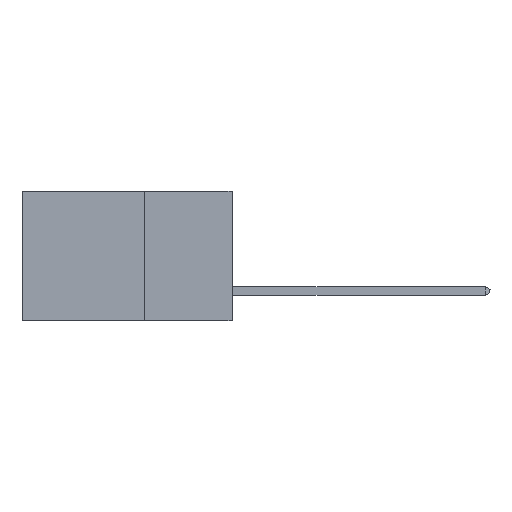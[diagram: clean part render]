
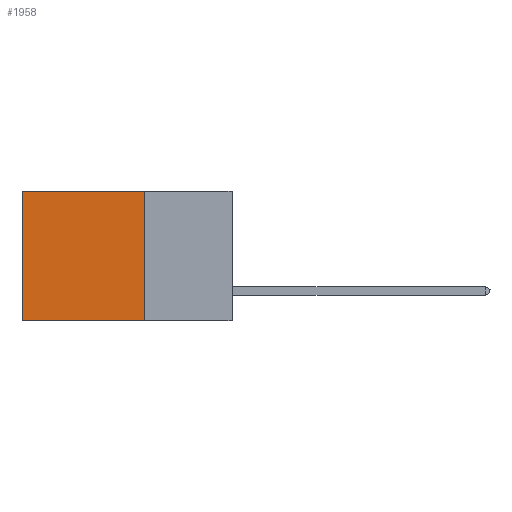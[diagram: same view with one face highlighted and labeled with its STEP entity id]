
A CAD part, left-side view. The second image highlights one B-rep face of the part: STEP entity #1958.
In plain terms, the highlighted planar face has unit normal (-1, 0, 0).
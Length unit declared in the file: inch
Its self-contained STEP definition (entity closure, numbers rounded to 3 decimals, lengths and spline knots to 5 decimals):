
#293 = DIRECTION ( 'NONE',  ( 1., 0., 0. ) ) ;
#711 = LINE ( 'NONE', #29720, #29429 ) ;
#1958 = ADVANCED_FACE ( 'NONE', ( #26955 ), #8711, .F. ) ;
#3336 = VERTEX_POINT ( 'NONE', #36147 ) ;
#3877 = EDGE_CURVE ( 'NONE', #3336, #5632, #28142, .T. ) ;
#5560 = LINE ( 'NONE', #17942, #28480 ) ;
#5632 = VERTEX_POINT ( 'NONE', #19012 ) ;
#5937 = CARTESIAN_POINT ( 'NONE',  ( 0.2875, 0.25, 0. ) ) ;
#6239 = EDGE_LOOP ( 'NONE', ( #8534, #12725, #10437, #15170 ) ) ;
#6482 = VECTOR ( 'NONE', #15194, 39.37008 ) ;
#6703 = EDGE_CURVE ( 'NONE', #11053, #5632, #16329, .T. ) ;
#8534 = ORIENTED_EDGE ( 'NONE', *, *, #6703, .T. ) ;
#8711 = PLANE ( 'NONE',  #30809 ) ;
#10437 = ORIENTED_EDGE ( 'NONE', *, *, #29652, .F. ) ;
#11053 = VERTEX_POINT ( 'NONE', #35909 ) ;
#12668 = CARTESIAN_POINT ( 'NONE',  ( 0.2875, 0.6, 0. ) ) ;
#12725 = ORIENTED_EDGE ( 'NONE', *, *, #3877, .F. ) ;
#14300 = VERTEX_POINT ( 'NONE', #24019 ) ;
#15170 = ORIENTED_EDGE ( 'NONE', *, *, #15172, .T. ) ;
#15172 = EDGE_CURVE ( 'NONE', #14300, #11053, #5560, .T. ) ;
#15194 = DIRECTION ( 'NONE',  ( 0., 1., 0. ) ) ;
#16329 = LINE ( 'NONE', #12668, #28453 ) ;
#17942 = CARTESIAN_POINT ( 'NONE',  ( 0.2875, 0.25, 0. ) ) ;
#18614 = CARTESIAN_POINT ( 'NONE',  ( 0.2875, 0.25, -0.37 ) ) ;
#18990 = DIRECTION ( 'NONE',  ( 0., 0., -1. ) ) ;
#19012 = CARTESIAN_POINT ( 'NONE',  ( 0.2875, 0.6, -0.37 ) ) ;
#21329 = DIRECTION ( 'NONE',  ( 0., 0., -1. ) ) ;
#24019 = CARTESIAN_POINT ( 'NONE',  ( 0.2875, 0.25, 0. ) ) ;
#26955 = FACE_OUTER_BOUND ( 'NONE', #6239, .T. ) ;
#27002 = DIRECTION ( 'NONE',  ( 0., 1., 0. ) ) ;
#28142 = LINE ( 'NONE', #18614, #6482 ) ;
#28453 = VECTOR ( 'NONE', #21329, 39.37008 ) ;
#28480 = VECTOR ( 'NONE', #27002, 39.37008 ) ;
#29429 = VECTOR ( 'NONE', #18990, 39.37008 ) ;
#29652 = EDGE_CURVE ( 'NONE', #14300, #3336, #711, .T. ) ;
#29720 = CARTESIAN_POINT ( 'NONE',  ( 0.2875, 0.25, 0. ) ) ;
#30809 = AXIS2_PLACEMENT_3D ( 'NONE', #5937, #293, #34785 ) ;
#34785 = DIRECTION ( 'NONE',  ( 0., 0., -1. ) ) ;
#35909 = CARTESIAN_POINT ( 'NONE',  ( 0.2875, 0.6, 0. ) ) ;
#36147 = CARTESIAN_POINT ( 'NONE',  ( 0.2875, 0.25, -0.37 ) ) ;
